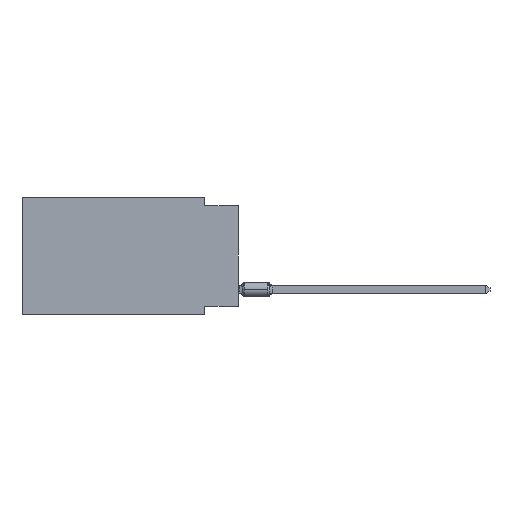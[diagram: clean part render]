
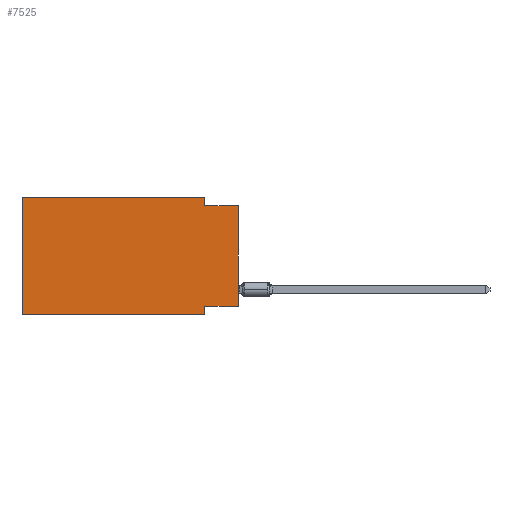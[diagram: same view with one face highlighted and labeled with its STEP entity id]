
A CAD part, left-side view. The second image highlights one B-rep face of the part: STEP entity #7525.
In plain terms, the highlighted planar face has unit normal (-1, 0, 0).
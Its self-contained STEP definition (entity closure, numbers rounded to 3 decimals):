
#190 = VECTOR ( 'NONE', #8882, 1000. ) ;
#548 = DIRECTION ( 'NONE',  ( 0., 0., 1. ) ) ;
#644 = DIRECTION ( 'NONE',  ( 0., 0., 1. ) ) ;
#939 = CARTESIAN_POINT ( 'NONE',  ( 0., 16.383, 0. ) ) ;
#987 = EDGE_CURVE ( 'NONE', #5319, #3005, #15457, .T. ) ;
#1384 = VECTOR ( 'NONE', #5360, 1000. ) ;
#1584 = CARTESIAN_POINT ( 'NONE',  ( 0., 2.54, 0. ) ) ;
#1752 = VERTEX_POINT ( 'NONE', #10354 ) ;
#1908 = CARTESIAN_POINT ( 'NONE',  ( 0., 0., -8.255 ) ) ;
#1956 = EDGE_LOOP ( 'NONE', ( #5899, #9917, #5861, #4630, #10937, #10183, #17085, #8500 ) ) ;
#1995 = CARTESIAN_POINT ( 'NONE',  ( 0., 2.54, -8.89 ) ) ;
#2294 = AXIS2_PLACEMENT_3D ( 'NONE', #939, #3504, #7527 ) ;
#2596 = EDGE_CURVE ( 'NONE', #17859, #8762, #16577, .T. ) ;
#3005 = VERTEX_POINT ( 'NONE', #9486 ) ;
#3504 = DIRECTION ( 'NONE',  ( 1., 0., 0. ) ) ;
#4004 = EDGE_CURVE ( 'NONE', #3005, #17767, #11178, .T. ) ;
#4346 = CARTESIAN_POINT ( 'NONE',  ( 0., 16.383, 0. ) ) ;
#4525 = CARTESIAN_POINT ( 'NONE',  ( 0., 2.54, -0.635 ) ) ;
#4630 = ORIENTED_EDGE ( 'NONE', *, *, #4004, .F. ) ;
#5083 = EDGE_CURVE ( 'NONE', #5319, #8341, #15036, .T. ) ;
#5144 = CARTESIAN_POINT ( 'NONE',  ( 0., 0., -0.635 ) ) ;
#5319 = VERTEX_POINT ( 'NONE', #6451 ) ;
#5360 = DIRECTION ( 'NONE',  ( 0., -1., 0. ) ) ;
#5597 = DIRECTION ( 'NONE',  ( 0., -1., 0. ) ) ;
#5861 = ORIENTED_EDGE ( 'NONE', *, *, #6630, .F. ) ;
#5899 = ORIENTED_EDGE ( 'NONE', *, *, #13143, .T. ) ;
#6072 = VECTOR ( 'NONE', #8920, 1000. ) ;
#6122 = DIRECTION ( 'NONE',  ( 0., 0., -1. ) ) ;
#6451 = CARTESIAN_POINT ( 'NONE',  ( 0., 16.383, -8.89 ) ) ;
#6477 = LINE ( 'NONE', #1995, #16828 ) ;
#6630 = EDGE_CURVE ( 'NONE', #17767, #17859, #17070, .T. ) ;
#7525 = ADVANCED_FACE ( 'NONE', ( #11640 ), #9150, .F. ) ;
#7527 = DIRECTION ( 'NONE',  ( 0., 0., -1. ) ) ;
#7624 = LINE ( 'NONE', #13204, #190 ) ;
#8341 = VERTEX_POINT ( 'NONE', #13410 ) ;
#8500 = ORIENTED_EDGE ( 'NONE', *, *, #12784, .F. ) ;
#8505 = LINE ( 'NONE', #14085, #13362 ) ;
#8762 = VERTEX_POINT ( 'NONE', #5144 ) ;
#8882 = DIRECTION ( 'NONE',  ( 0., 1., 0. ) ) ;
#8920 = DIRECTION ( 'NONE',  ( 0., 0., -1. ) ) ;
#9150 = PLANE ( 'NONE',  #2294 ) ;
#9486 = CARTESIAN_POINT ( 'NONE',  ( 0., 16.383, 0. ) ) ;
#9917 = ORIENTED_EDGE ( 'NONE', *, *, #2596, .F. ) ;
#10183 = ORIENTED_EDGE ( 'NONE', *, *, #5083, .T. ) ;
#10236 = VERTEX_POINT ( 'NONE', #1908 ) ;
#10354 = CARTESIAN_POINT ( 'NONE',  ( 0., 2.54, -8.255 ) ) ;
#10828 = EDGE_CURVE ( 'NONE', #1752, #8341, #6477, .T. ) ;
#10937 = ORIENTED_EDGE ( 'NONE', *, *, #987, .F. ) ;
#11074 = CARTESIAN_POINT ( 'NONE',  ( 0., 0., -0.635 ) ) ;
#11178 = LINE ( 'NONE', #4346, #17557 ) ;
#11508 = CARTESIAN_POINT ( 'NONE',  ( 0., 16.383, 0. ) ) ;
#11640 = FACE_OUTER_BOUND ( 'NONE', #1956, .T. ) ;
#12784 = EDGE_CURVE ( 'NONE', #10236, #1752, #7624, .T. ) ;
#13143 = EDGE_CURVE ( 'NONE', #10236, #8762, #8505, .T. ) ;
#13204 = CARTESIAN_POINT ( 'NONE',  ( 0., 0., -8.255 ) ) ;
#13362 = VECTOR ( 'NONE', #644, 1000. ) ;
#13410 = CARTESIAN_POINT ( 'NONE',  ( 0., 2.54, -8.89 ) ) ;
#13897 = VECTOR ( 'NONE', #548, 1000. ) ;
#14085 = CARTESIAN_POINT ( 'NONE',  ( 0., 0., 0. ) ) ;
#14483 = VECTOR ( 'NONE', #5597, 1000. ) ;
#15036 = LINE ( 'NONE', #17889, #1384 ) ;
#15457 = LINE ( 'NONE', #11508, #13897 ) ;
#16577 = LINE ( 'NONE', #11074, #14483 ) ;
#16828 = VECTOR ( 'NONE', #6122, 1000. ) ;
#16959 = DIRECTION ( 'NONE',  ( 0., -1., 0. ) ) ;
#17070 = LINE ( 'NONE', #17268, #6072 ) ;
#17085 = ORIENTED_EDGE ( 'NONE', *, *, #10828, .F. ) ;
#17268 = CARTESIAN_POINT ( 'NONE',  ( 0., 2.54, 0. ) ) ;
#17557 = VECTOR ( 'NONE', #16959, 1000. ) ;
#17767 = VERTEX_POINT ( 'NONE', #1584 ) ;
#17859 = VERTEX_POINT ( 'NONE', #4525 ) ;
#17889 = CARTESIAN_POINT ( 'NONE',  ( 0., 16.383, -8.89 ) ) ;
